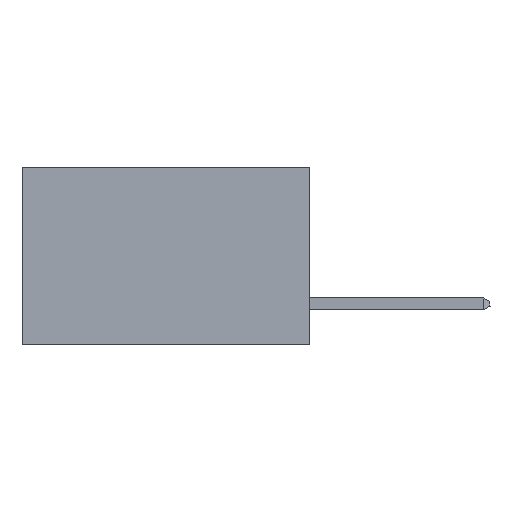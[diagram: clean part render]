
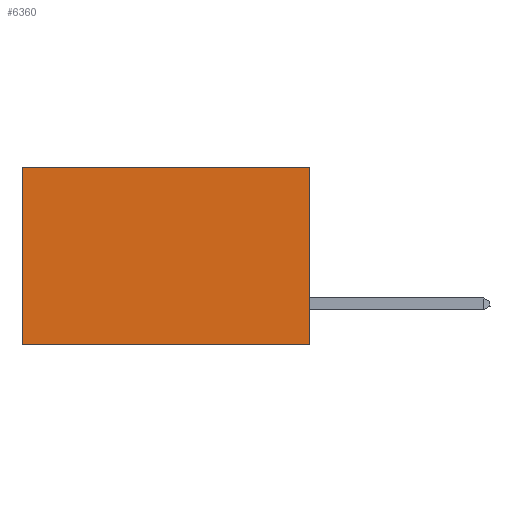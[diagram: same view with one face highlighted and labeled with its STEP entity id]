
A CAD part, left-side view. The second image highlights one B-rep face of the part: STEP entity #6360.
In plain terms, the highlighted planar face has unit normal (-1, 0, 0).
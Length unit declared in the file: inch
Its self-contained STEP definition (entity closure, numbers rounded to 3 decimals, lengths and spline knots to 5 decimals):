
#547 = VERTEX_POINT ( 'NONE', #6506 ) ;
#706 = EDGE_LOOP ( 'NONE', ( #4235, #38972, #23867, #33743 ) ) ;
#1074 = DIRECTION ( 'NONE',  ( 1., 0., 0. ) ) ;
#1136 = CARTESIAN_POINT ( 'NONE',  ( 0.2875, 0., -0.37 ) ) ;
#3188 = DIRECTION ( 'NONE',  ( 0., 0., -1. ) ) ;
#4235 = ORIENTED_EDGE ( 'NONE', *, *, #36065, .T. ) ;
#5031 = CARTESIAN_POINT ( 'NONE',  ( 0.2875, 0., 0. ) ) ;
#6360 = ADVANCED_FACE ( 'NONE', ( #20819 ), #19558, .F. ) ;
#6506 = CARTESIAN_POINT ( 'NONE',  ( 0.2875, 0.6, -0.37 ) ) ;
#6647 = LINE ( 'NONE', #18590, #30324 ) ;
#8047 = LINE ( 'NONE', #5031, #39882 ) ;
#8078 = CARTESIAN_POINT ( 'NONE',  ( 0.2875, 0., 0. ) ) ;
#9994 = CARTESIAN_POINT ( 'NONE',  ( 0.2875, 0., -0.37 ) ) ;
#10393 = EDGE_CURVE ( 'NONE', #36495, #16375, #17657, .T. ) ;
#11261 = DIRECTION ( 'NONE',  ( 0., 1., 0. ) ) ;
#14137 = EDGE_CURVE ( 'NONE', #16375, #547, #34537, .T. ) ;
#14750 = VECTOR ( 'NONE', #34694, 39.37008 ) ;
#16375 = VERTEX_POINT ( 'NONE', #1136 ) ;
#17657 = LINE ( 'NONE', #26807, #25832 ) ;
#18590 = CARTESIAN_POINT ( 'NONE',  ( 0.2875, 0.6, 0. ) ) ;
#19558 = PLANE ( 'NONE',  #33198 ) ;
#20819 = FACE_OUTER_BOUND ( 'NONE', #706, .T. ) ;
#21515 = CARTESIAN_POINT ( 'NONE',  ( 0.2875, 0.6, 0. ) ) ;
#23867 = ORIENTED_EDGE ( 'NONE', *, *, #10393, .F. ) ;
#25832 = VECTOR ( 'NONE', #33421, 39.37008 ) ;
#26807 = CARTESIAN_POINT ( 'NONE',  ( 0.2875, 0., 0. ) ) ;
#28185 = DIRECTION ( 'NONE',  ( 0., 0., -1. ) ) ;
#28957 = EDGE_CURVE ( 'NONE', #36495, #38305, #8047, .T. ) ;
#30324 = VECTOR ( 'NONE', #3188, 39.37008 ) ;
#33198 = AXIS2_PLACEMENT_3D ( 'NONE', #34538, #1074, #28185 ) ;
#33421 = DIRECTION ( 'NONE',  ( 0., 0., -1. ) ) ;
#33743 = ORIENTED_EDGE ( 'NONE', *, *, #28957, .T. ) ;
#34537 = LINE ( 'NONE', #9994, #14750 ) ;
#34538 = CARTESIAN_POINT ( 'NONE',  ( 0.2875, 0., 0. ) ) ;
#34694 = DIRECTION ( 'NONE',  ( 0., 1., 0. ) ) ;
#36065 = EDGE_CURVE ( 'NONE', #38305, #547, #6647, .T. ) ;
#36495 = VERTEX_POINT ( 'NONE', #8078 ) ;
#38305 = VERTEX_POINT ( 'NONE', #21515 ) ;
#38972 = ORIENTED_EDGE ( 'NONE', *, *, #14137, .F. ) ;
#39882 = VECTOR ( 'NONE', #11261, 39.37008 ) ;
